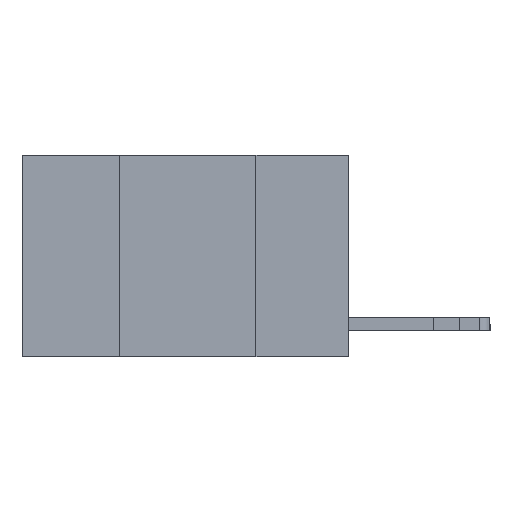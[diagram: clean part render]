
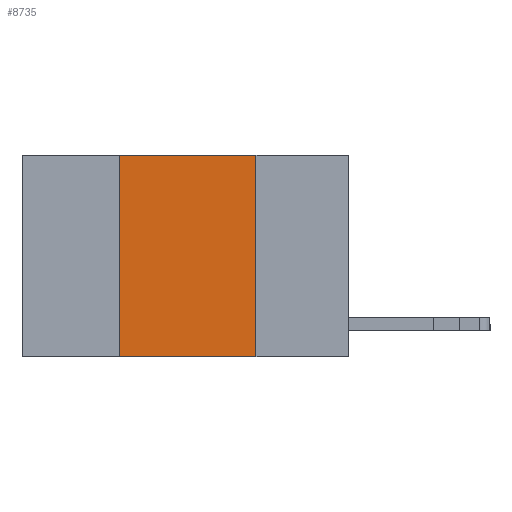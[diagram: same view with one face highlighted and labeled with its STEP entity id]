
A CAD part, left-side view. The second image highlights one B-rep face of the part: STEP entity #8735.
In plain terms, the highlighted planar face has unit normal (-1, 0, 0).
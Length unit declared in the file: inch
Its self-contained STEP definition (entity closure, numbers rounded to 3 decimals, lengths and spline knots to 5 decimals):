
#125 = CARTESIAN_POINT ( 'NONE',  ( 0., 0.42, -0.37 ) ) ;
#363 = CARTESIAN_POINT ( 'NONE',  ( 0., 0.17, -0.37 ) ) ;
#1675 = VERTEX_POINT ( 'NONE', #125 ) ;
#1682 = LINE ( 'NONE', #11686, #7840 ) ;
#1735 = VECTOR ( 'NONE', #14835, 39.37008 ) ;
#2043 = AXIS2_PLACEMENT_3D ( 'NONE', #5646, #12202, #19097 ) ;
#2429 = EDGE_CURVE ( 'NONE', #7784, #19370, #1682, .T. ) ;
#3120 = CARTESIAN_POINT ( 'NONE',  ( 0., 0.17, 0. ) ) ;
#4347 = CARTESIAN_POINT ( 'NONE',  ( 0., 0.42, 0. ) ) ;
#5646 = CARTESIAN_POINT ( 'NONE',  ( 0., 0.6, 0. ) ) ;
#6423 = LINE ( 'NONE', #8457, #1735 ) ;
#7784 = VERTEX_POINT ( 'NONE', #16347 ) ;
#7840 = VECTOR ( 'NONE', #19784, 39.37008 ) ;
#8117 = VECTOR ( 'NONE', #10878, 39.37008 ) ;
#8456 = ORIENTED_EDGE ( 'NONE', *, *, #8533, .T. ) ;
#8457 = CARTESIAN_POINT ( 'NONE',  ( 0., 0.17, 0. ) ) ;
#8533 = EDGE_CURVE ( 'NONE', #1675, #19827, #18229, .T. ) ;
#8735 = ADVANCED_FACE ( 'NONE', ( #20393 ), #12512, .F. ) ;
#9697 = LINE ( 'NONE', #4347, #8117 ) ;
#9812 = EDGE_CURVE ( 'NONE', #19370, #19827, #6423, .T. ) ;
#10878 = DIRECTION ( 'NONE',  ( 0., 0., 1. ) ) ;
#11686 = CARTESIAN_POINT ( 'NONE',  ( 0., 0.6, 0. ) ) ;
#12202 = DIRECTION ( 'NONE',  ( 1., 0., 0. ) ) ;
#12444 = EDGE_LOOP ( 'NONE', ( #14800, #18834, #14973, #8456 ) ) ;
#12512 = PLANE ( 'NONE',  #2043 ) ;
#13385 = CARTESIAN_POINT ( 'NONE',  ( 0., 0.6, -0.37 ) ) ;
#14800 = ORIENTED_EDGE ( 'NONE', *, *, #9812, .F. ) ;
#14835 = DIRECTION ( 'NONE',  ( 0., 0., -1. ) ) ;
#14973 = ORIENTED_EDGE ( 'NONE', *, *, #20041, .F. ) ;
#15798 = VECTOR ( 'NONE', #16396, 39.37008 ) ;
#16347 = CARTESIAN_POINT ( 'NONE',  ( 0., 0.42, 0. ) ) ;
#16396 = DIRECTION ( 'NONE',  ( 0., -1., 0. ) ) ;
#18229 = LINE ( 'NONE', #13385, #15798 ) ;
#18834 = ORIENTED_EDGE ( 'NONE', *, *, #2429, .F. ) ;
#19097 = DIRECTION ( 'NONE',  ( 0., 0., -1. ) ) ;
#19370 = VERTEX_POINT ( 'NONE', #3120 ) ;
#19784 = DIRECTION ( 'NONE',  ( 0., -1., 0. ) ) ;
#19827 = VERTEX_POINT ( 'NONE', #363 ) ;
#20041 = EDGE_CURVE ( 'NONE', #1675, #7784, #9697, .T. ) ;
#20393 = FACE_OUTER_BOUND ( 'NONE', #12444, .T. ) ;
